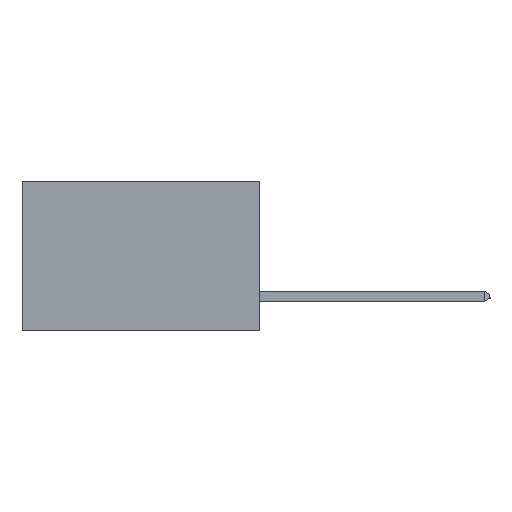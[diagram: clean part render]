
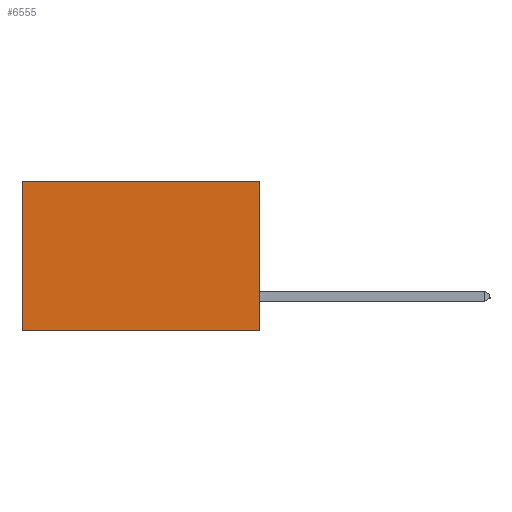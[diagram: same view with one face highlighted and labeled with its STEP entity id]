
A CAD part, left-side view. The second image highlights one B-rep face of the part: STEP entity #6555.
In plain terms, the highlighted planar face has unit normal (-1, 0, 0).
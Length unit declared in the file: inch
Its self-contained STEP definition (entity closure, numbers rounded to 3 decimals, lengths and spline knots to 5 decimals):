
#270 = EDGE_LOOP ( 'NONE', ( #9707, #8567, #11362, #7206 ) ) ;
#1097 = FACE_OUTER_BOUND ( 'NONE', #270, .T. ) ;
#1815 = VECTOR ( 'NONE', #9743, 39.37008 ) ;
#2216 = DIRECTION ( 'NONE',  ( 0., 0., -1. ) ) ;
#2229 = VERTEX_POINT ( 'NONE', #10576 ) ;
#2748 = LINE ( 'NONE', #5801, #13847 ) ;
#2900 = CARTESIAN_POINT ( 'NONE',  ( 0.277, 0., -0.37 ) ) ;
#3070 = VERTEX_POINT ( 'NONE', #8268 ) ;
#3648 = DIRECTION ( 'NONE',  ( 0., 0., -1. ) ) ;
#3667 = DIRECTION ( 'NONE',  ( 1., 0., 0. ) ) ;
#3691 = CARTESIAN_POINT ( 'NONE',  ( 0.277, 0., -0.37 ) ) ;
#3775 = PLANE ( 'NONE',  #6439 ) ;
#3927 = VERTEX_POINT ( 'NONE', #10561 ) ;
#5801 = CARTESIAN_POINT ( 'NONE',  ( 0.277, 0., 0. ) ) ;
#6439 = AXIS2_PLACEMENT_3D ( 'NONE', #3691, #3667, #3648 ) ;
#6487 = DIRECTION ( 'NONE',  ( 0., 1., 0. ) ) ;
#6555 = ADVANCED_FACE ( 'NONE', ( #1097 ), #3775, .F. ) ;
#6760 = LINE ( 'NONE', #2900, #12048 ) ;
#7206 = ORIENTED_EDGE ( 'NONE', *, *, #7907, .T. ) ;
#7342 = EDGE_CURVE ( 'NONE', #2229, #3070, #13394, .T. ) ;
#7907 = EDGE_CURVE ( 'NONE', #2229, #3927, #2748, .T. ) ;
#8268 = CARTESIAN_POINT ( 'NONE',  ( 0.277, 0., -0.37 ) ) ;
#8567 = ORIENTED_EDGE ( 'NONE', *, *, #11164, .F. ) ;
#9707 = ORIENTED_EDGE ( 'NONE', *, *, #10782, .T. ) ;
#9729 = CARTESIAN_POINT ( 'NONE',  ( 0.277, 0., -0.37 ) ) ;
#9743 = DIRECTION ( 'NONE',  ( 0., 0., -1. ) ) ;
#10396 = CARTESIAN_POINT ( 'NONE',  ( 0.277, 0.59, -0.37 ) ) ;
#10434 = VERTEX_POINT ( 'NONE', #10396 ) ;
#10561 = CARTESIAN_POINT ( 'NONE',  ( 0.277, 0.59, 0. ) ) ;
#10576 = CARTESIAN_POINT ( 'NONE',  ( 0.277, 0., 0. ) ) ;
#10782 = EDGE_CURVE ( 'NONE', #3927, #10434, #11742, .T. ) ;
#11164 = EDGE_CURVE ( 'NONE', #3070, #10434, #6760, .T. ) ;
#11362 = ORIENTED_EDGE ( 'NONE', *, *, #7342, .F. ) ;
#11593 = DIRECTION ( 'NONE',  ( 0., 1., 0. ) ) ;
#11742 = LINE ( 'NONE', #13040, #14120 ) ;
#12048 = VECTOR ( 'NONE', #11593, 39.37008 ) ;
#13040 = CARTESIAN_POINT ( 'NONE',  ( 0.277, 0.59, -0.37 ) ) ;
#13394 = LINE ( 'NONE', #9729, #1815 ) ;
#13847 = VECTOR ( 'NONE', #6487, 39.37008 ) ;
#14120 = VECTOR ( 'NONE', #2216, 39.37008 ) ;
